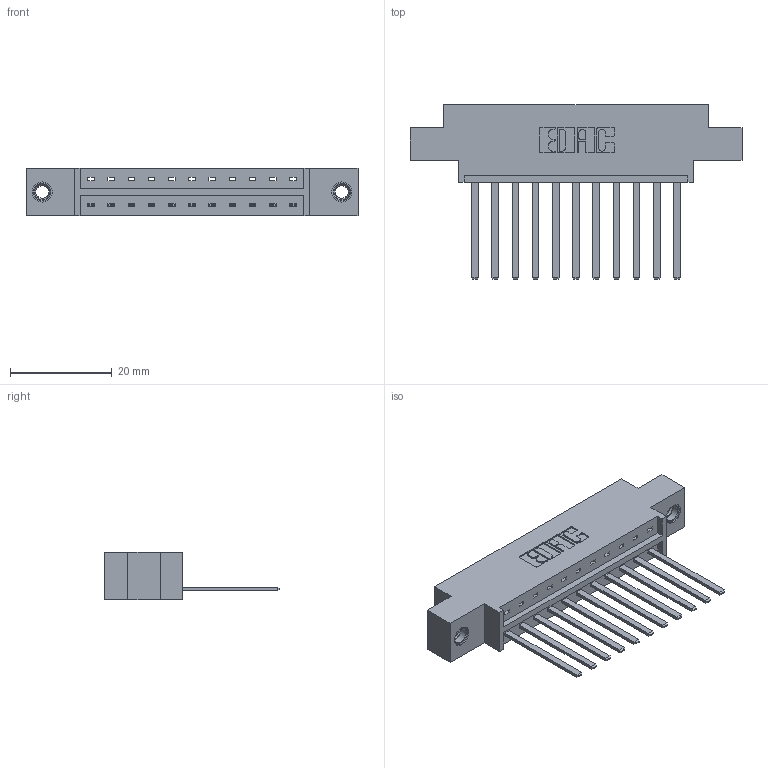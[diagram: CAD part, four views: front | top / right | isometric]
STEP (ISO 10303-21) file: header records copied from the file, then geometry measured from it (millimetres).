
FILE_DESCRIPTION (( 'STEP AP203' ), '1' );
FILE_NAME ('333-011-544-607.STEP', '2018-07-31T23:38:48', ( '' ), ( '' ), 'SwSTEP 2.0', 'SolidWorks 2016', '' );
FILE_SCHEMA (( 'CONFIG_CONTROL_DESIGN' ));
Length unit declared in the file: inch
Products named in the file (4): 333 Part_Offset - .156 Dia - TI; 345-292-001_345-293-144; 345-250-001_345-250-005-103; 333-011-544-607
Assembly tree (14 placements, depth 2):
  333-011-544-607
    333 Part_Offset - .156 Dia - TI
    345-292-001_345-293-144  x11
    345-250-001_345-250-005-103  x2
Bounding box: 65.13 x 34.3 x 9.4 mm (x, y, z)
Volume: 6173 mm3; surface area: 7125.9 mm2
Topology: 14 solids, 14 shells, 750 faces, 2197 edges, 1442 vertices
Faces by surface type: plane 524, cylinder 210, cone 12, torus 4
Entity records: 11868 total; most frequent: CARTESIAN_POINT 2034, ORIENTED_EDGE 1974, DIRECTION 1807, EDGE_CURVE 987, VECTOR 843, LINE 843, VERTEX_POINT 652, AXIS2_PLACEMENT_3D 482
